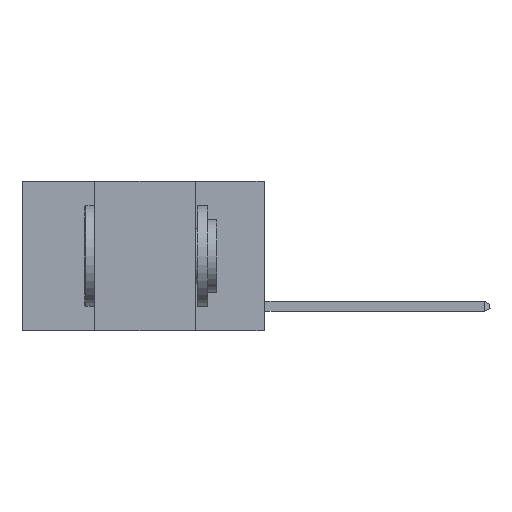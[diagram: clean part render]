
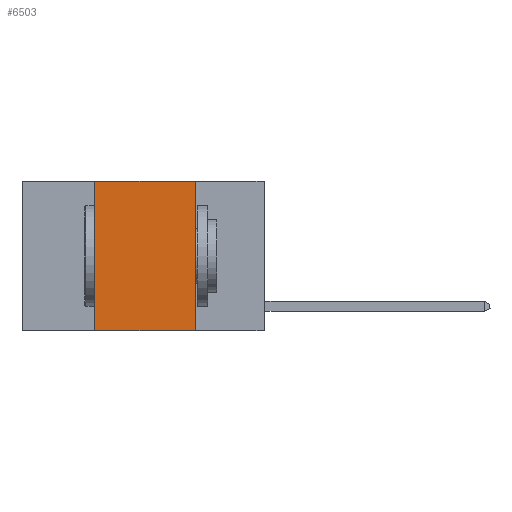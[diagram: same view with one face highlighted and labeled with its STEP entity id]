
A CAD part, left-side view. The second image highlights one B-rep face of the part: STEP entity #6503.
In plain terms, the highlighted planar face has unit normal (-1, 0, 0).
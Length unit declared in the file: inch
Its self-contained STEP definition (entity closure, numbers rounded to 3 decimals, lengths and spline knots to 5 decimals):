
#14 = EDGE_CURVE ( 'NONE', #12559, #11135, #20380, .T. ) ;
#239 = CARTESIAN_POINT ( 'NONE',  ( 0., 0.6, -0.37 ) ) ;
#694 = FACE_OUTER_BOUND ( 'NONE', #7935, .T. ) ;
#1333 = VECTOR ( 'NONE', #10161, 39.37008 ) ;
#2270 = ORIENTED_EDGE ( 'NONE', *, *, #9964, .F. ) ;
#3599 = DIRECTION ( 'NONE',  ( 0., 0., -1. ) ) ;
#3800 = DIRECTION ( 'NONE',  ( 0., 0., -1. ) ) ;
#5207 = EDGE_CURVE ( 'NONE', #19685, #11135, #15468, .T. ) ;
#5506 = VERTEX_POINT ( 'NONE', #10114 ) ;
#5801 = DIRECTION ( 'NONE',  ( 1., 0., 0. ) ) ;
#6043 = ORIENTED_EDGE ( 'NONE', *, *, #14, .F. ) ;
#6193 = VECTOR ( 'NONE', #7041, 39.37008 ) ;
#6503 = ADVANCED_FACE ( 'NONE', ( #694 ), #12473, .F. ) ;
#7041 = DIRECTION ( 'NONE',  ( 0., -1., 0. ) ) ;
#7116 = DIRECTION ( 'NONE',  ( 0., -1., 0. ) ) ;
#7314 = AXIS2_PLACEMENT_3D ( 'NONE', #12698, #5801, #3800 ) ;
#7935 = EDGE_LOOP ( 'NONE', ( #6043, #11939, #2270, #20993 ) ) ;
#8664 = LINE ( 'NONE', #15553, #15493 ) ;
#9943 = CARTESIAN_POINT ( 'NONE',  ( 0., 0.42, 0. ) ) ;
#9964 = EDGE_CURVE ( 'NONE', #19685, #5506, #11818, .T. ) ;
#10114 = CARTESIAN_POINT ( 'NONE',  ( 0., 0.42, 0. ) ) ;
#10161 = DIRECTION ( 'NONE',  ( 0., 0., 1. ) ) ;
#10451 = VECTOR ( 'NONE', #3599, 39.37008 ) ;
#11135 = VERTEX_POINT ( 'NONE', #20368 ) ;
#11818 = LINE ( 'NONE', #9943, #1333 ) ;
#11939 = ORIENTED_EDGE ( 'NONE', *, *, #19439, .F. ) ;
#12473 = PLANE ( 'NONE',  #7314 ) ;
#12559 = VERTEX_POINT ( 'NONE', #14881 ) ;
#12698 = CARTESIAN_POINT ( 'NONE',  ( 0., 0.6, 0. ) ) ;
#14881 = CARTESIAN_POINT ( 'NONE',  ( 0., 0.17, 0. ) ) ;
#15468 = LINE ( 'NONE', #239, #6193 ) ;
#15493 = VECTOR ( 'NONE', #7116, 39.37008 ) ;
#15553 = CARTESIAN_POINT ( 'NONE',  ( 0., 0.6, 0. ) ) ;
#18583 = CARTESIAN_POINT ( 'NONE',  ( 0., 0.17, 0. ) ) ;
#19439 = EDGE_CURVE ( 'NONE', #5506, #12559, #8664, .T. ) ;
#19685 = VERTEX_POINT ( 'NONE', #21726 ) ;
#20368 = CARTESIAN_POINT ( 'NONE',  ( 0., 0.17, -0.37 ) ) ;
#20380 = LINE ( 'NONE', #18583, #10451 ) ;
#20993 = ORIENTED_EDGE ( 'NONE', *, *, #5207, .T. ) ;
#21726 = CARTESIAN_POINT ( 'NONE',  ( 0., 0.42, -0.37 ) ) ;
